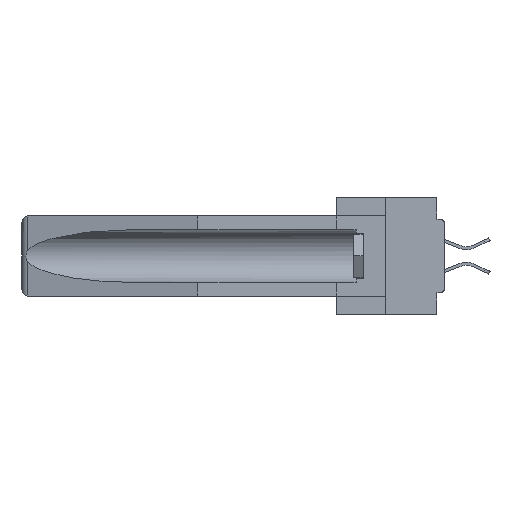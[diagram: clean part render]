
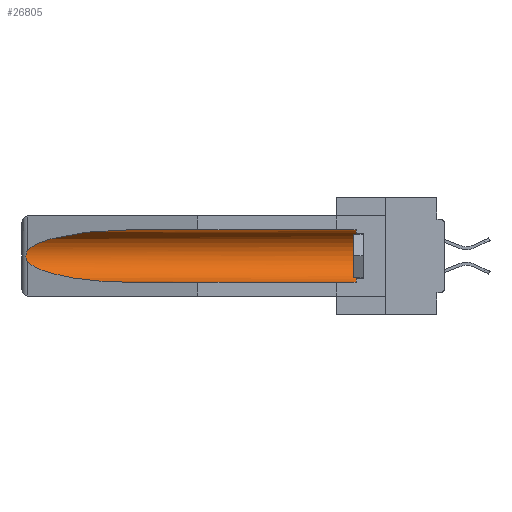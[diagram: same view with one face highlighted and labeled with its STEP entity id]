
A CAD part, left-side view. The second image highlights one B-rep face of the part: STEP entity #26805.
In plain terms, the highlighted cylindrical face has radius 2.857 mm (diameter 5.715 mm), a partial arc.
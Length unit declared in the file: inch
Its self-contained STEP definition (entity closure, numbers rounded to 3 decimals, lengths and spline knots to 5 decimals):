
#392 = AXIS2_PLACEMENT_3D ( 'NONE', #12568, #27044, #5698 ) ;
#1460 = ORIENTED_EDGE ( 'NONE', *, *, #24185, .T. ) ;
#2091 = EDGE_CURVE ( 'NONE', #41774, #20913, #39186, .T. ) ;
#4390 = DIRECTION ( 'NONE',  ( 0., 1., 0. ) ) ;
#4631 = DIRECTION ( 'NONE',  ( 0., 1., 0. ) ) ;
#5698 = DIRECTION ( 'NONE',  ( 0., 0., 1. ) ) ;
#5914 = ORIENTED_EDGE ( 'NONE', *, *, #41640, .T. ) ;
#8801 = CARTESIAN_POINT ( 'NONE',  ( 0.26537, 1.52718, -0.19328 ) ) ;
#9408 = CARTESIAN_POINT ( 'NONE',  ( 0.26537, 1.52718, -0.19328 ) ) ;
#10613 = ORIENTED_EDGE ( 'NONE', *, *, #2091, .T. ) ;
#11870 = CARTESIAN_POINT ( 'NONE',  ( 0.26654, 1.53092, -0.15636 ) ) ;
#12349 = CARTESIAN_POINT ( 'NONE',  ( 0.155, 0.126, -0.284 ) ) ;
#12568 = CARTESIAN_POINT ( 'NONE',  ( 0.155, 0.126, -0.1715 ) ) ;
#12792 = CARTESIAN_POINT ( 'NONE',  ( 0.155, 0.126, -0.059 ) ) ;
#13091 = CIRCLE ( 'NONE', #392, 0.1125 ) ;
#15227 = CARTESIAN_POINT ( 'NONE',  ( 0.155, 1.07973, -0.059 ) ) ;
#15319 = CARTESIAN_POINT ( 'NONE',  ( 0.2675, 1.53308, -0.16763 ) ) ;
#16610 = DIRECTION ( 'NONE',  ( 0., 1., 0. ) ) ;
#18132 = CARTESIAN_POINT ( 'NONE',  ( 0.25451, 1.48313, -0.24835 ) ) ;
#18995 = CARTESIAN_POINT ( 'NONE',  ( 0.26655, 1.53094, -0.18657 ) ) ;
#19684 = CARTESIAN_POINT ( 'NONE',  ( 0.155, -0.30754, -0.284 ) ) ;
#20421 = CARTESIAN_POINT ( 'NONE',  ( 0.26537, 1.52718, -0.14972 ) ) ;
#20552 =( BOUNDED_CURVE ( )  B_SPLINE_CURVE ( 3, ( #24568, #24865, #34946, #35397 ),
 .UNSPECIFIED., .F., .F. ) 
 B_SPLINE_CURVE_WITH_KNOTS ( ( 4, 4 ),
 ( 4.71239, 6.08839 ),
 .UNSPECIFIED. ) 
 CURVE ( )  GEOMETRIC_REPRESENTATION_ITEM ( )  RATIONAL_B_SPLINE_CURVE ( ( 1., 0.848, 0.848, 1. ) ) 
 REPRESENTATION_ITEM ( '' )  );
#20825 = VECTOR ( 'NONE', #16610, 39.37008 ) ;
#20913 = VERTEX_POINT ( 'NONE', #15227 ) ;
#21144 = EDGE_CURVE ( 'NONE', #24960, #29446, #35039, .T. ) ;
#22525 = CARTESIAN_POINT ( 'NONE',  ( 0.26597, 1.5296, -0.19026 ) ) ;
#22562 = EDGE_LOOP ( 'NONE', ( #5914, #1460, #42793, #40324, #22853, #10613 ) ) ;
#22853 = ORIENTED_EDGE ( 'NONE', *, *, #27011, .T. ) ;
#22989 = CARTESIAN_POINT ( 'NONE',  ( 0.26597, 1.52961, -0.15275 ) ) ;
#23933 = B_SPLINE_CURVE_WITH_KNOTS ( 'NONE', 3,
 ( #25872, #22989, #11870, #36300, #15319, #39777, #32938, #18995, #22525, #9408 ),
 .UNSPECIFIED., .F., .F.,
 ( 4, 2, 2, 2, 4 ),
 ( 0., 0.00029, 0.00058, 0.00087, 0.00117 ),
 .UNSPECIFIED. ) ;
#24185 = EDGE_CURVE ( 'NONE', #30063, #30356, #23933, .T. ) ;
#24568 = CARTESIAN_POINT ( 'NONE',  ( 0.155, 1.07973, -0.059 ) ) ;
#24865 = CARTESIAN_POINT ( 'NONE',  ( 0.21114, 1.30732, -0.059 ) ) ;
#24960 = VERTEX_POINT ( 'NONE', #12349 ) ;
#25872 = CARTESIAN_POINT ( 'NONE',  ( 0.26537, 1.52718, -0.14972 ) ) ;
#26727 =( BOUNDED_CURVE ( )  B_SPLINE_CURVE ( 3, ( #35873, #18132, #28989, #36192 ),
 .UNSPECIFIED., .F., .F. ) 
 B_SPLINE_CURVE_WITH_KNOTS ( ( 4, 4 ),
 ( 0.1948, 1.5708 ),
 .UNSPECIFIED. ) 
 CURVE ( )  GEOMETRIC_REPRESENTATION_ITEM ( )  RATIONAL_B_SPLINE_CURVE ( ( 1., 0.848, 0.848, 1. ) ) 
 REPRESENTATION_ITEM ( '' )  );
#26805 = ADVANCED_FACE ( 'NONE', ( #31840 ), #38914, .F. ) ;
#27011 = EDGE_CURVE ( 'NONE', #24960, #41774, #13091, .T. ) ;
#27044 = DIRECTION ( 'NONE',  ( 0., -1., 0. ) ) ;
#28750 = DIRECTION ( 'NONE',  ( 0., 0., 1. ) ) ;
#28989 = CARTESIAN_POINT ( 'NONE',  ( 0.21114, 1.30732, -0.284 ) ) ;
#29446 = VERTEX_POINT ( 'NONE', #36306 ) ;
#30063 = VERTEX_POINT ( 'NONE', #20421 ) ;
#30356 = VERTEX_POINT ( 'NONE', #8801 ) ;
#31840 = FACE_OUTER_BOUND ( 'NONE', #22562, .T. ) ;
#32118 = CARTESIAN_POINT ( 'NONE',  ( 0.155, -0.30754, -0.1715 ) ) ;
#32938 = CARTESIAN_POINT ( 'NONE',  ( 0.2673, 1.53269, -0.17917 ) ) ;
#34946 = CARTESIAN_POINT ( 'NONE',  ( 0.25451, 1.48313, -0.09465 ) ) ;
#35039 = LINE ( 'NONE', #19684, #20825 ) ;
#35397 = CARTESIAN_POINT ( 'NONE',  ( 0.26537, 1.52718, -0.14972 ) ) ;
#35873 = CARTESIAN_POINT ( 'NONE',  ( 0.26537, 1.52718, -0.19328 ) ) ;
#36192 = CARTESIAN_POINT ( 'NONE',  ( 0.155, 1.07973, -0.284 ) ) ;
#36300 = CARTESIAN_POINT ( 'NONE',  ( 0.2673, 1.5327, -0.16383 ) ) ;
#36306 = CARTESIAN_POINT ( 'NONE',  ( 0.155, 1.07973, -0.284 ) ) ;
#38458 = AXIS2_PLACEMENT_3D ( 'NONE', #32118, #4631, #28750 ) ;
#38914 = CYLINDRICAL_SURFACE ( 'NONE', #38458, 0.1125 ) ;
#39034 = CARTESIAN_POINT ( 'NONE',  ( 0.155, -0.30754, -0.059 ) ) ;
#39186 = LINE ( 'NONE', #39034, #40322 ) ;
#39777 = CARTESIAN_POINT ( 'NONE',  ( 0.2675, 1.53308, -0.17534 ) ) ;
#40322 = VECTOR ( 'NONE', #4390, 39.37008 ) ;
#40324 = ORIENTED_EDGE ( 'NONE', *, *, #21144, .F. ) ;
#41640 = EDGE_CURVE ( 'NONE', #20913, #30063, #20552, .T. ) ;
#41719 = EDGE_CURVE ( 'NONE', #30356, #29446, #26727, .T. ) ;
#41774 = VERTEX_POINT ( 'NONE', #12792 ) ;
#42793 = ORIENTED_EDGE ( 'NONE', *, *, #41719, .T. ) ;
